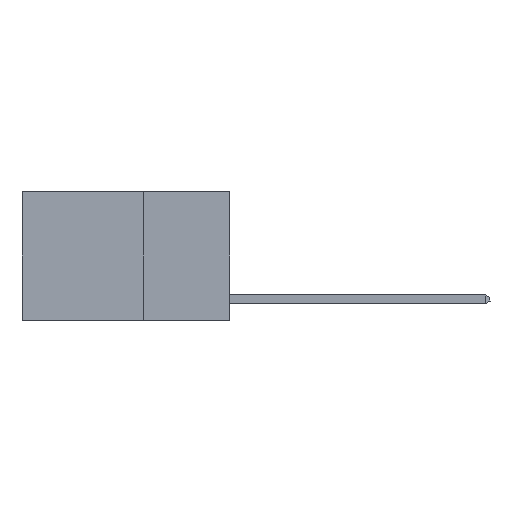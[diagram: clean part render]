
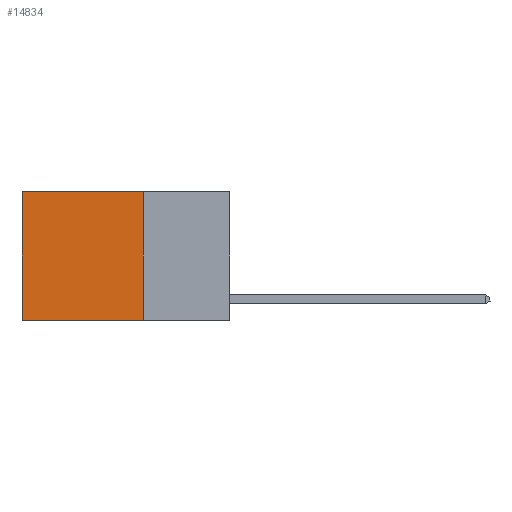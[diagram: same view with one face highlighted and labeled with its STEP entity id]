
A CAD part, left-side view. The second image highlights one B-rep face of the part: STEP entity #14834.
In plain terms, the highlighted planar face has unit normal (-1, 0, 0).
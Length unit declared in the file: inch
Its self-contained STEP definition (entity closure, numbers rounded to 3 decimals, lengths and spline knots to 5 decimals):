
#660 = DIRECTION ( 'NONE',  ( 0., 0., -1. ) ) ;
#2337 = ORIENTED_EDGE ( 'NONE', *, *, #5314, .F. ) ;
#3418 = VERTEX_POINT ( 'NONE', #24375 ) ;
#3936 = CARTESIAN_POINT ( 'NONE',  ( 0.2625, 0.25, 0. ) ) ;
#4198 = VERTEX_POINT ( 'NONE', #19245 ) ;
#4253 = LINE ( 'NONE', #12659, #20667 ) ;
#4335 = DIRECTION ( 'NONE',  ( 0., 0., -1. ) ) ;
#4553 = VECTOR ( 'NONE', #18206, 39.37008 ) ;
#5071 = DIRECTION ( 'NONE',  ( 0., 1., 0. ) ) ;
#5314 = EDGE_CURVE ( 'NONE', #4198, #3418, #16348, .T. ) ;
#5466 = CARTESIAN_POINT ( 'NONE',  ( 0.2625, 0.6, -0.37 ) ) ;
#7348 = CARTESIAN_POINT ( 'NONE',  ( 0.2625, 0.6, 0. ) ) ;
#7814 = PLANE ( 'NONE',  #18499 ) ;
#7997 = ORIENTED_EDGE ( 'NONE', *, *, #9768, .F. ) ;
#9768 = EDGE_CURVE ( 'NONE', #3418, #16383, #20406, .T. ) ;
#10442 = DIRECTION ( 'NONE',  ( 0., 0., -1. ) ) ;
#12520 = FACE_OUTER_BOUND ( 'NONE', #15712, .T. ) ;
#12659 = CARTESIAN_POINT ( 'NONE',  ( 0.2625, 0.6, 0. ) ) ;
#14098 = ORIENTED_EDGE ( 'NONE', *, *, #16171, .T. ) ;
#14834 = ADVANCED_FACE ( 'NONE', ( #12520 ), #7814, .F. ) ;
#15712 = EDGE_LOOP ( 'NONE', ( #14098, #7997, #2337, #22311 ) ) ;
#16171 = EDGE_CURVE ( 'NONE', #16737, #16383, #4253, .T. ) ;
#16247 = DIRECTION ( 'NONE',  ( 1., 0., 0. ) ) ;
#16348 = LINE ( 'NONE', #3936, #18426 ) ;
#16383 = VERTEX_POINT ( 'NONE', #5466 ) ;
#16432 = EDGE_CURVE ( 'NONE', #4198, #16737, #26181, .T. ) ;
#16737 = VERTEX_POINT ( 'NONE', #7348 ) ;
#18206 = DIRECTION ( 'NONE',  ( 0., 1., 0. ) ) ;
#18426 = VECTOR ( 'NONE', #4335, 39.37008 ) ;
#18499 = AXIS2_PLACEMENT_3D ( 'NONE', #20948, #16247, #10442 ) ;
#19245 = CARTESIAN_POINT ( 'NONE',  ( 0.2625, 0.25, 0. ) ) ;
#19348 = VECTOR ( 'NONE', #5071, 39.37008 ) ;
#20406 = LINE ( 'NONE', #26776, #4553 ) ;
#20667 = VECTOR ( 'NONE', #660, 39.37008 ) ;
#20948 = CARTESIAN_POINT ( 'NONE',  ( 0.2625, 0.25, 0. ) ) ;
#22311 = ORIENTED_EDGE ( 'NONE', *, *, #16432, .T. ) ;
#24375 = CARTESIAN_POINT ( 'NONE',  ( 0.2625, 0.25, -0.37 ) ) ;
#26049 = CARTESIAN_POINT ( 'NONE',  ( 0.2625, 0.25, 0. ) ) ;
#26181 = LINE ( 'NONE', #26049, #19348 ) ;
#26776 = CARTESIAN_POINT ( 'NONE',  ( 0.2625, 0.25, -0.37 ) ) ;
